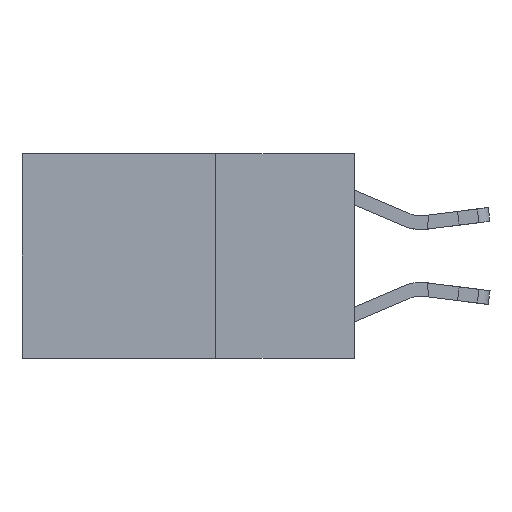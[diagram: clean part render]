
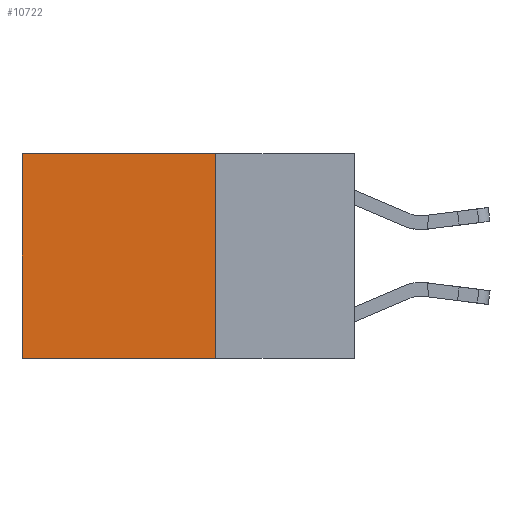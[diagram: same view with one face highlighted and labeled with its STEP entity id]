
A CAD part, left-side view. The second image highlights one B-rep face of the part: STEP entity #10722.
In plain terms, the highlighted planar face has unit normal (-1, 0, 0).
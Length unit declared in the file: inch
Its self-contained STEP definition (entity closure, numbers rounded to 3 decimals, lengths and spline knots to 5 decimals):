
#178 = EDGE_CURVE ( 'NONE', #13256, #8464, #3786, .T. ) ;
#306 = AXIS2_PLACEMENT_3D ( 'NONE', #16132, #2357, #12051 ) ;
#376 = LINE ( 'NONE', #6596, #7357 ) ;
#1260 = LINE ( 'NONE', #12852, #15993 ) ;
#2357 = DIRECTION ( 'NONE',  ( 1., 0., 0. ) ) ;
#2482 = CARTESIAN_POINT ( 'NONE',  ( 0.2625, 0.6, -0.37 ) ) ;
#2544 = EDGE_CURVE ( 'NONE', #3424, #8464, #7782, .T. ) ;
#2547 = EDGE_CURVE ( 'NONE', #13007, #3424, #376, .T. ) ;
#3424 = VERTEX_POINT ( 'NONE', #15629 ) ;
#3571 = ORIENTED_EDGE ( 'NONE', *, *, #2547, .F. ) ;
#3786 = LINE ( 'NONE', #13416, #14375 ) ;
#4201 = ORIENTED_EDGE ( 'NONE', *, *, #178, .T. ) ;
#4597 = DIRECTION ( 'NONE',  ( 0., 1., 0. ) ) ;
#5106 = PLANE ( 'NONE',  #306 ) ;
#5124 = FACE_OUTER_BOUND ( 'NONE', #15650, .T. ) ;
#6596 = CARTESIAN_POINT ( 'NONE',  ( 0.2625, 0.25, 0. ) ) ;
#7357 = VECTOR ( 'NONE', #7988, 39.37008 ) ;
#7782 = LINE ( 'NONE', #14821, #14704 ) ;
#7988 = DIRECTION ( 'NONE',  ( 0., 0., -1. ) ) ;
#8464 = VERTEX_POINT ( 'NONE', #2482 ) ;
#10722 = ADVANCED_FACE ( 'NONE', ( #5124 ), #5106, .F. ) ;
#10759 = ORIENTED_EDGE ( 'NONE', *, *, #2544, .F. ) ;
#11770 = ORIENTED_EDGE ( 'NONE', *, *, #13470, .T. ) ;
#11800 = DIRECTION ( 'NONE',  ( 0., 0., -1. ) ) ;
#12051 = DIRECTION ( 'NONE',  ( 0., 0., -1. ) ) ;
#12852 = CARTESIAN_POINT ( 'NONE',  ( 0.2625, 0.25, 0. ) ) ;
#13007 = VERTEX_POINT ( 'NONE', #13234 ) ;
#13234 = CARTESIAN_POINT ( 'NONE',  ( 0.2625, 0.25, 0. ) ) ;
#13256 = VERTEX_POINT ( 'NONE', #16511 ) ;
#13416 = CARTESIAN_POINT ( 'NONE',  ( 0.2625, 0.6, 0. ) ) ;
#13470 = EDGE_CURVE ( 'NONE', #13007, #13256, #1260, .T. ) ;
#13491 = DIRECTION ( 'NONE',  ( 0., 1., 0. ) ) ;
#14375 = VECTOR ( 'NONE', #11800, 39.37008 ) ;
#14704 = VECTOR ( 'NONE', #13491, 39.37008 ) ;
#14821 = CARTESIAN_POINT ( 'NONE',  ( 0.2625, 0.25, -0.37 ) ) ;
#15629 = CARTESIAN_POINT ( 'NONE',  ( 0.2625, 0.25, -0.37 ) ) ;
#15650 = EDGE_LOOP ( 'NONE', ( #4201, #10759, #3571, #11770 ) ) ;
#15993 = VECTOR ( 'NONE', #4597, 39.37008 ) ;
#16132 = CARTESIAN_POINT ( 'NONE',  ( 0.2625, 0.25, 0. ) ) ;
#16511 = CARTESIAN_POINT ( 'NONE',  ( 0.2625, 0.6, 0. ) ) ;
